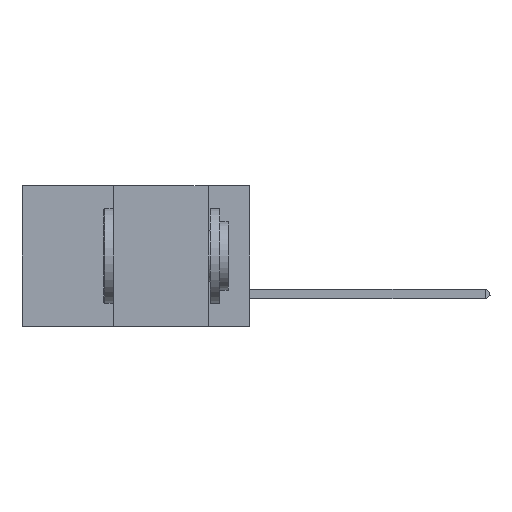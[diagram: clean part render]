
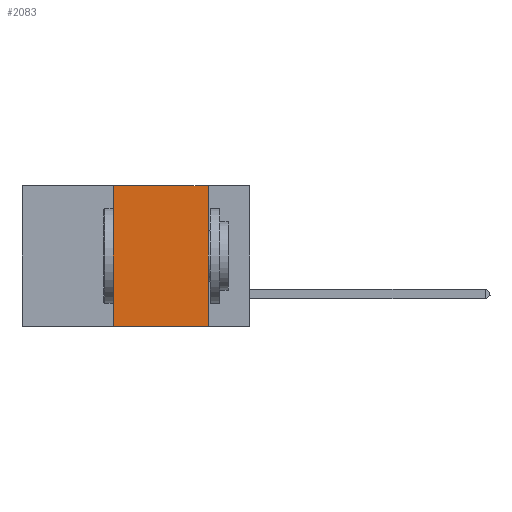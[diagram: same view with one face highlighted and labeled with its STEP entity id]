
A CAD part, left-side view. The second image highlights one B-rep face of the part: STEP entity #2083.
In plain terms, the highlighted planar face has unit normal (-1, 0, 0).
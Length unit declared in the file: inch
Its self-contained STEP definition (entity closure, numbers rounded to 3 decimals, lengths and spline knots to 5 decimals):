
#165 = VERTEX_POINT ( 'NONE', #6842 ) ;
#310 = DIRECTION ( 'NONE',  ( 1., 0., 0. ) ) ;
#1168 = DIRECTION ( 'NONE',  ( 0., -1., 0. ) ) ;
#1655 = VECTOR ( 'NONE', #1168, 39.37008 ) ;
#2083 = ADVANCED_FACE ( 'NONE', ( #4772 ), #2671, .F. ) ;
#2293 = CARTESIAN_POINT ( 'NONE',  ( 0., 0.36, -0.37 ) ) ;
#2671 = PLANE ( 'NONE',  #25103 ) ;
#3354 = VECTOR ( 'NONE', #5306, 39.37008 ) ;
#3461 = EDGE_LOOP ( 'NONE', ( #23054, #21857, #24986, #11654 ) ) ;
#4772 = FACE_OUTER_BOUND ( 'NONE', #3461, .T. ) ;
#5158 = VERTEX_POINT ( 'NONE', #10000 ) ;
#5306 = DIRECTION ( 'NONE',  ( 0., 0., -1. ) ) ;
#6842 = CARTESIAN_POINT ( 'NONE',  ( 0., 0.11, 0. ) ) ;
#6887 = VERTEX_POINT ( 'NONE', #2293 ) ;
#8381 = CARTESIAN_POINT ( 'NONE',  ( 0., 0.11, -0.37 ) ) ;
#8998 = LINE ( 'NONE', #13886, #17632 ) ;
#10000 = CARTESIAN_POINT ( 'NONE',  ( 0., 0.36, 0. ) ) ;
#11654 = ORIENTED_EDGE ( 'NONE', *, *, #12352, .T. ) ;
#11844 = EDGE_CURVE ( 'NONE', #6887, #5158, #16173, .T. ) ;
#12352 = EDGE_CURVE ( 'NONE', #6887, #20489, #25208, .T. ) ;
#13886 = CARTESIAN_POINT ( 'NONE',  ( 0., 0.6, 0. ) ) ;
#16137 = EDGE_CURVE ( 'NONE', #165, #20489, #25778, .T. ) ;
#16173 = LINE ( 'NONE', #24723, #17614 ) ;
#16650 = CARTESIAN_POINT ( 'NONE',  ( 0., 0.6, 0. ) ) ;
#17614 = VECTOR ( 'NONE', #22398, 39.37008 ) ;
#17632 = VECTOR ( 'NONE', #25361, 39.37008 ) ;
#18770 = DIRECTION ( 'NONE',  ( 0., 0., -1. ) ) ;
#20489 = VERTEX_POINT ( 'NONE', #8381 ) ;
#21857 = ORIENTED_EDGE ( 'NONE', *, *, #28120, .F. ) ;
#22398 = DIRECTION ( 'NONE',  ( 0., 0., 1. ) ) ;
#23054 = ORIENTED_EDGE ( 'NONE', *, *, #16137, .F. ) ;
#23389 = CARTESIAN_POINT ( 'NONE',  ( 0., 0.11, 0. ) ) ;
#24723 = CARTESIAN_POINT ( 'NONE',  ( 0., 0.36, 0. ) ) ;
#24986 = ORIENTED_EDGE ( 'NONE', *, *, #11844, .F. ) ;
#25103 = AXIS2_PLACEMENT_3D ( 'NONE', #16650, #310, #18770 ) ;
#25208 = LINE ( 'NONE', #26869, #1655 ) ;
#25361 = DIRECTION ( 'NONE',  ( 0., -1., 0. ) ) ;
#25778 = LINE ( 'NONE', #23389, #3354 ) ;
#26869 = CARTESIAN_POINT ( 'NONE',  ( 0., 0.6, -0.37 ) ) ;
#28120 = EDGE_CURVE ( 'NONE', #5158, #165, #8998, .T. ) ;
